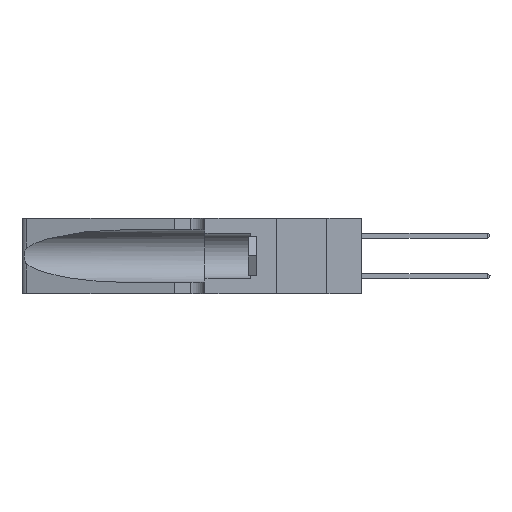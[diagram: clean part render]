
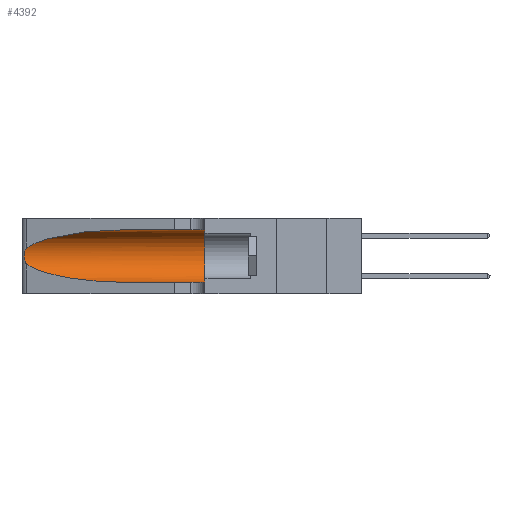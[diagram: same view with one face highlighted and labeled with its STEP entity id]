
A CAD part, left-side view. The second image highlights one B-rep face of the part: STEP entity #4392.
In plain terms, the highlighted cylindrical face has radius 3.308 mm (diameter 6.617 mm), a partial arc.
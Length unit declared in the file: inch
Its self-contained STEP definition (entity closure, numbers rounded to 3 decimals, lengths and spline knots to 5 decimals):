
#338 = CARTESIAN_POINT ( 'NONE',  ( 0.25787, 1.23484, 0.2124 ) ) ;
#523 = CARTESIAN_POINT ( 'NONE',  ( 0.1305, 0.72297, 0.05475 ) ) ;
#2082 = EDGE_CURVE ( 'NONE', #44719, #29607, #25259, .T. ) ;
#2251 = B_SPLINE_CURVE_WITH_KNOTS ( 'NONE', 3,
 ( #35508, #28425, #21490, #338, #25062, #3923, #28568, #7453, #32106, #11009, #35650, #14560, #39217, #18074 ),
 .UNSPECIFIED., .F., .F.,
 ( 4, 2, 2, 2, 2, 2, 4 ),
 ( 0., 0.00027, 0.00053, 0.00107, 0.0016, 0.00187, 0.00214 ),
 .UNSPECIFIED. ) ;
#2309 = CIRCLE ( 'NONE', #8488, 0.13025 ) ;
#2727 = CARTESIAN_POINT ( 'NONE',  ( 0.1305, 1.61858, 0.05475 ) ) ;
#3403 = CARTESIAN_POINT ( 'NONE',  ( 0.2373, 1.15595, 0.28018 ) ) ;
#3407 = CARTESIAN_POINT ( 'NONE',  ( 0.1305, 1.61858, 0.31525 ) ) ;
#3923 = CARTESIAN_POINT ( 'NONE',  ( 0.26018, 1.23835, 0.19895 ) ) ;
#4090 = EDGE_LOOP ( 'NONE', ( #45494, #23476, #11416, #42586, #27231, #43751 ) ) ;
#4336 = VERTEX_POINT ( 'NONE', #523 ) ;
#4392 = ADVANCED_FACE ( 'NONE', ( #19976 ), #9493, .F. ) ;
#4671 = CARTESIAN_POINT ( 'NONE',  ( 0.1305, 0.35, 0.05475 ) ) ;
#5742 = CARTESIAN_POINT ( 'NONE',  ( 0.2373, 1.15595, 0.08982 ) ) ;
#6083 = DIRECTION ( 'NONE',  ( 0., -1., 0. ) ) ;
#7453 = CARTESIAN_POINT ( 'NONE',  ( 0.26075, 1.23896, 0.178 ) ) ;
#7932 = DIRECTION ( 'NONE',  ( 0., -1., 0. ) ) ;
#8326 = EDGE_CURVE ( 'NONE', #10739, #4336, #43196, .T. ) ;
#8488 = AXIS2_PLACEMENT_3D ( 'NONE', #20809, #45436, #24388 ) ;
#8717 = VECTOR ( 'NONE', #6083, 39.37008 ) ;
#9248 = CARTESIAN_POINT ( 'NONE',  ( 0.1305, 0.72297, 0.05475 ) ) ;
#9493 = CYLINDRICAL_SURFACE ( 'NONE', #31288, 0.13025 ) ;
#10739 = VERTEX_POINT ( 'NONE', #29941 ) ;
#11009 = CARTESIAN_POINT ( 'NONE',  ( 0.25856, 1.23593, 0.16098 ) ) ;
#11416 = ORIENTED_EDGE ( 'NONE', *, *, #8326, .T. ) ;
#14560 = CARTESIAN_POINT ( 'NONE',  ( 0.25639, 1.23186, 0.15144 ) ) ;
#15831 = VECTOR ( 'NONE', #28028, 39.37008 ) ;
#16304 = EDGE_CURVE ( 'NONE', #44719, #21539, #18585, .T. ) ;
#17103 = EDGE_CURVE ( 'NONE', #21539, #10739, #2251, .T. ) ;
#18074 = CARTESIAN_POINT ( 'NONE',  ( 0.25487, 1.22718, 0.14631 ) ) ;
#18585 =( BOUNDED_CURVE ( )  B_SPLINE_CURVE ( 3, ( #24518, #45576, #3403, #28026 ),
 .UNSPECIFIED., .F., .F. ) 
 B_SPLINE_CURVE_WITH_KNOTS ( ( 4, 4 ),
 ( 1.5708, 2.84003 ),
 .UNSPECIFIED. ) 
 CURVE ( )  GEOMETRIC_REPRESENTATION_ITEM ( )  RATIONAL_B_SPLINE_CURVE ( ( 1., 0.87, 0.87, 1. ) ) 
 REPRESENTATION_ITEM ( '' )  );
#19189 = LINE ( 'NONE', #2727, #8717 ) ;
#19976 = FACE_OUTER_BOUND ( 'NONE', #4090, .T. ) ;
#20809 = CARTESIAN_POINT ( 'NONE',  ( 0.1305, 0.35, 0.185 ) ) ;
#21490 = CARTESIAN_POINT ( 'NONE',  ( 0.25639, 1.23184, 0.21858 ) ) ;
#21539 = VERTEX_POINT ( 'NONE', #31322 ) ;
#21981 = CARTESIAN_POINT ( 'NONE',  ( 0.1305, 1.61858, 0.185 ) ) ;
#22441 = VERTEX_POINT ( 'NONE', #4671 ) ;
#23476 = ORIENTED_EDGE ( 'NONE', *, *, #17103, .T. ) ;
#24388 = DIRECTION ( 'NONE',  ( 0., 0., 1. ) ) ;
#24518 = CARTESIAN_POINT ( 'NONE',  ( 0.1305, 0.72297, 0.31525 ) ) ;
#25062 = CARTESIAN_POINT ( 'NONE',  ( 0.25854, 1.2359, 0.20912 ) ) ;
#25259 = LINE ( 'NONE', #3407, #15831 ) ;
#26862 = CARTESIAN_POINT ( 'NONE',  ( 0.25487, 1.22718, 0.14631 ) ) ;
#27231 = ORIENTED_EDGE ( 'NONE', *, *, #40950, .F. ) ;
#28026 = CARTESIAN_POINT ( 'NONE',  ( 0.25487, 1.22718, 0.22369 ) ) ;
#28028 = DIRECTION ( 'NONE',  ( 0., -1., 0. ) ) ;
#28425 = CARTESIAN_POINT ( 'NONE',  ( 0.25555, 1.22994, 0.2215 ) ) ;
#28568 = CARTESIAN_POINT ( 'NONE',  ( 0.26075, 1.23896, 0.19203 ) ) ;
#29006 = EDGE_CURVE ( 'NONE', #4336, #22441, #19189, .T. ) ;
#29607 = VERTEX_POINT ( 'NONE', #30511 ) ;
#29941 = CARTESIAN_POINT ( 'NONE',  ( 0.25487, 1.22718, 0.14631 ) ) ;
#30377 = CARTESIAN_POINT ( 'NONE',  ( 0.18966, 0.96281, 0.05475 ) ) ;
#30511 = CARTESIAN_POINT ( 'NONE',  ( 0.1305, 0.35, 0.31525 ) ) ;
#31288 = AXIS2_PLACEMENT_3D ( 'NONE', #21981, #7932, #39552 ) ;
#31322 = CARTESIAN_POINT ( 'NONE',  ( 0.25487, 1.22718, 0.22369 ) ) ;
#32106 = CARTESIAN_POINT ( 'NONE',  ( 0.26017, 1.23833, 0.17102 ) ) ;
#35508 = CARTESIAN_POINT ( 'NONE',  ( 0.25487, 1.22718, 0.22369 ) ) ;
#35650 = CARTESIAN_POINT ( 'NONE',  ( 0.25789, 1.23486, 0.15765 ) ) ;
#39217 = CARTESIAN_POINT ( 'NONE',  ( 0.25555, 1.22993, 0.14849 ) ) ;
#39552 = DIRECTION ( 'NONE',  ( 0., 0., -1. ) ) ;
#40950 = EDGE_CURVE ( 'NONE', #29607, #22441, #2309, .T. ) ;
#41881 = CARTESIAN_POINT ( 'NONE',  ( 0.1305, 0.72297, 0.31525 ) ) ;
#42586 = ORIENTED_EDGE ( 'NONE', *, *, #29006, .T. ) ;
#43196 =( BOUNDED_CURVE ( )  B_SPLINE_CURVE ( 3, ( #26862, #5742, #30377, #9248 ),
 .UNSPECIFIED., .F., .F. ) 
 B_SPLINE_CURVE_WITH_KNOTS ( ( 4, 4 ),
 ( 3.44316, 4.71239 ),
 .UNSPECIFIED. ) 
 CURVE ( )  GEOMETRIC_REPRESENTATION_ITEM ( )  RATIONAL_B_SPLINE_CURVE ( ( 1., 0.87, 0.87, 1. ) ) 
 REPRESENTATION_ITEM ( '' )  );
#43751 = ORIENTED_EDGE ( 'NONE', *, *, #2082, .F. ) ;
#44719 = VERTEX_POINT ( 'NONE', #41881 ) ;
#45436 = DIRECTION ( 'NONE',  ( 0., 1., 0. ) ) ;
#45494 = ORIENTED_EDGE ( 'NONE', *, *, #16304, .T. ) ;
#45576 = CARTESIAN_POINT ( 'NONE',  ( 0.18966, 0.96281, 0.31525 ) ) ;
